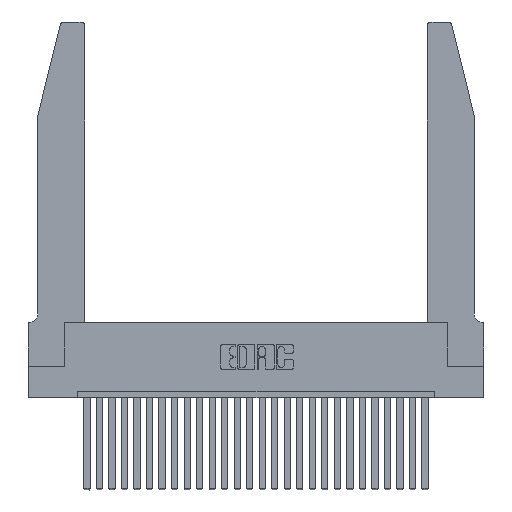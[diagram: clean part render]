
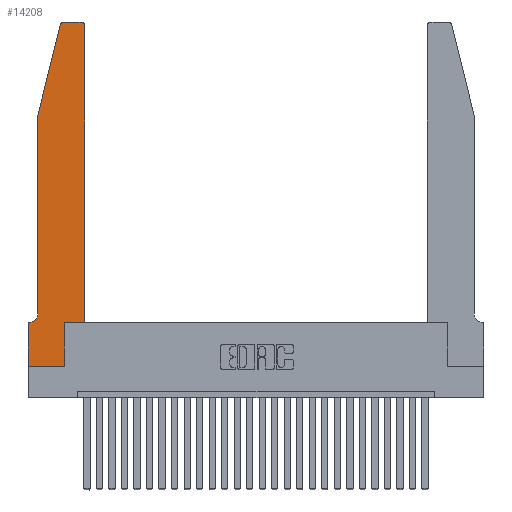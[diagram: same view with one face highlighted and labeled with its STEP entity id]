
A CAD part, top view. The second image highlights one B-rep face of the part: STEP entity #14208.
In plain terms, the highlighted planar face has unit normal (0, 0, 1).
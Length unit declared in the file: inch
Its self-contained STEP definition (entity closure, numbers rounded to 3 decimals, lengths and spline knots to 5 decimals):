
#185 = DIRECTION ( 'NONE',  ( 1., 0., 0. ) ) ;
#214 = ORIENTED_EDGE ( 'NONE', *, *, #17555, .T. ) ;
#443 = VECTOR ( 'NONE', #8880, 39.37008 ) ;
#586 = CARTESIAN_POINT ( 'NONE',  ( 0.2605, 2.75, 0.37 ) ) ;
#982 = EDGE_CURVE ( 'NONE', #19145, #22454, #14397, .T. ) ;
#1420 = EDGE_CURVE ( 'NONE', #19592, #8688, #21034, .T. ) ;
#1856 = AXIS2_PLACEMENT_3D ( 'NONE', #17353, #21535, #23645 ) ;
#1897 = CARTESIAN_POINT ( 'NONE',  ( 0.2865, 0.35, 0.37 ) ) ;
#2103 = CARTESIAN_POINT ( 'NONE',  ( 0.0055, 0.35, 0.37 ) ) ;
#2295 = VECTOR ( 'NONE', #12975, 39.37008 ) ;
#2397 = FACE_OUTER_BOUND ( 'NONE', #25852, .T. ) ;
#3489 = ORIENTED_EDGE ( 'NONE', *, *, #18303, .T. ) ;
#3810 = CIRCLE ( 'NONE', #1856, 0.03 ) ;
#4190 = LINE ( 'NONE', #22873, #16880 ) ;
#4228 = EDGE_CURVE ( 'NONE', #26464, #13652, #11018, .T. ) ;
#4322 = CARTESIAN_POINT ( 'NONE',  ( 0.4205, 2.75, 0.37 ) ) ;
#4453 = ORIENTED_EDGE ( 'NONE', *, *, #21800, .T. ) ;
#4820 = DIRECTION ( 'NONE',  ( -1., 0., 0. ) ) ;
#4891 = ORIENTED_EDGE ( 'NONE', *, *, #11842, .T. ) ;
#4965 = DIRECTION ( 'NONE',  ( 0., 1., 0. ) ) ;
#5534 = CARTESIAN_POINT ( 'NONE',  ( 0.4505, 2.72, 0.37 ) ) ;
#6410 = CARTESIAN_POINT ( 'NONE',  ( 0., 0., 0.37 ) ) ;
#6593 = CARTESIAN_POINT ( 'NONE',  ( 0.0755, 2., 0.37 ) ) ;
#6822 = LINE ( 'NONE', #22109, #26061 ) ;
#6920 = CIRCLE ( 'NONE', #12871, 0.07 ) ;
#7059 = EDGE_CURVE ( 'NONE', #15594, #19592, #4190, .T. ) ;
#7537 = LINE ( 'NONE', #1897, #22514 ) ;
#7857 = CARTESIAN_POINT ( 'NONE',  ( 0.4205, 2.72, 0.37 ) ) ;
#8307 = VERTEX_POINT ( 'NONE', #15370 ) ;
#8688 = VERTEX_POINT ( 'NONE', #20620 ) ;
#8880 = DIRECTION ( 'NONE',  ( -1., 0., 0. ) ) ;
#9003 = ORIENTED_EDGE ( 'NONE', *, *, #1420, .T. ) ;
#9033 = PLANE ( 'NONE',  #21551 ) ;
#9568 = LINE ( 'NONE', #10798, #11600 ) ;
#10331 = EDGE_CURVE ( 'NONE', #17383, #26464, #17255, .T. ) ;
#10453 = CARTESIAN_POINT ( 'NONE',  ( 0.2865, 0.35, 0.37 ) ) ;
#10753 = DIRECTION ( 'NONE',  ( 0., -1., 0. ) ) ;
#10798 = CARTESIAN_POINT ( 'NONE',  ( 0.4505, 0.35, 0.37 ) ) ;
#11018 = LINE ( 'NONE', #586, #25864 ) ;
#11600 = VECTOR ( 'NONE', #185, 39.37008 ) ;
#11688 = CARTESIAN_POINT ( 'NONE',  ( 0., 0.35, 0.37 ) ) ;
#11842 = EDGE_CURVE ( 'NONE', #8688, #12333, #7537, .T. ) ;
#11906 = DIRECTION ( 'NONE',  ( 0., 0., 1. ) ) ;
#12333 = VERTEX_POINT ( 'NONE', #10453 ) ;
#12681 = LINE ( 'NONE', #19303, #2295 ) ;
#12753 = VECTOR ( 'NONE', #10753, 39.37008 ) ;
#12871 = AXIS2_PLACEMENT_3D ( 'NONE', #15538, #19623, #23682 ) ;
#12975 = DIRECTION ( 'NONE',  ( -0.239, -0.971, 0. ) ) ;
#13126 = DIRECTION ( 'NONE',  ( 0., 0., 1. ) ) ;
#13652 = VERTEX_POINT ( 'NONE', #23832 ) ;
#13680 = CARTESIAN_POINT ( 'NONE',  ( 0.0755, 2., 0.37 ) ) ;
#14208 = ADVANCED_FACE ( 'NONE', ( #2397 ), #9033, .T. ) ;
#14397 = LINE ( 'NONE', #6593, #12753 ) ;
#14686 = DIRECTION ( 'NONE',  ( 0., 1., 0. ) ) ;
#15370 = CARTESIAN_POINT ( 'NONE',  ( 0.4505, 0.35, 0.37 ) ) ;
#15371 = VECTOR ( 'NONE', #18825, 39.37008 ) ;
#15538 = CARTESIAN_POINT ( 'NONE',  ( 0.0055, 0.42, 0.37 ) ) ;
#15594 = VERTEX_POINT ( 'NONE', #11688 ) ;
#15820 = EDGE_CURVE ( 'NONE', #22454, #16036, #6920, .T. ) ;
#16036 = VERTEX_POINT ( 'NONE', #2103 ) ;
#16338 = DIRECTION ( 'NONE',  ( 1., 0., 0. ) ) ;
#16537 = AXIS2_PLACEMENT_3D ( 'NONE', #7857, #11906, #16338 ) ;
#16880 = VECTOR ( 'NONE', #22963, 39.37008 ) ;
#17255 = CIRCLE ( 'NONE', #16537, 0.03 ) ;
#17298 = DIRECTION ( 'NONE',  ( 1., 0., 0. ) ) ;
#17353 = CARTESIAN_POINT ( 'NONE',  ( 0.284, 2.72, 0.37 ) ) ;
#17383 = VERTEX_POINT ( 'NONE', #5534 ) ;
#17555 = EDGE_CURVE ( 'NONE', #8307, #17383, #6822, .T. ) ;
#17819 = ORIENTED_EDGE ( 'NONE', *, *, #982, .T. ) ;
#17975 = CARTESIAN_POINT ( 'NONE',  ( 0.25487, 2.72718, 0.37 ) ) ;
#18303 = EDGE_CURVE ( 'NONE', #16036, #15594, #18473, .T. ) ;
#18473 = LINE ( 'NONE', #19433, #443 ) ;
#18825 = DIRECTION ( 'NONE',  ( 1., 0., 0. ) ) ;
#19145 = VERTEX_POINT ( 'NONE', #13680 ) ;
#19303 = CARTESIAN_POINT ( 'NONE',  ( 0.0755, 2., 0.37 ) ) ;
#19433 = CARTESIAN_POINT ( 'NONE',  ( 0.0755, 0.35, 0.37 ) ) ;
#19592 = VERTEX_POINT ( 'NONE', #24529 ) ;
#19617 = CARTESIAN_POINT ( 'NONE',  ( 0., 0.35, 0.37 ) ) ;
#19623 = DIRECTION ( 'NONE',  ( 0., 0., -1. ) ) ;
#20620 = CARTESIAN_POINT ( 'NONE',  ( 0.2865, 0., 0.37 ) ) ;
#20985 = ORIENTED_EDGE ( 'NONE', *, *, #7059, .T. ) ;
#21034 = LINE ( 'NONE', #6410, #15371 ) ;
#21535 = DIRECTION ( 'NONE',  ( 0., 0., 1. ) ) ;
#21551 = AXIS2_PLACEMENT_3D ( 'NONE', #19617, #13126, #17298 ) ;
#21681 = CARTESIAN_POINT ( 'NONE',  ( 0.0755, 0.42, 0.37 ) ) ;
#21800 = EDGE_CURVE ( 'NONE', #13652, #26780, #3810, .T. ) ;
#22109 = CARTESIAN_POINT ( 'NONE',  ( 0.4505, 0.35, 0.37 ) ) ;
#22454 = VERTEX_POINT ( 'NONE', #21681 ) ;
#22514 = VECTOR ( 'NONE', #14686, 39.37008 ) ;
#22873 = CARTESIAN_POINT ( 'NONE',  ( 0., 0., 0.37 ) ) ;
#22963 = DIRECTION ( 'NONE',  ( 0., -1., 0. ) ) ;
#23157 = ORIENTED_EDGE ( 'NONE', *, *, #15820, .T. ) ;
#23645 = DIRECTION ( 'NONE',  ( 1., 0., 0. ) ) ;
#23682 = DIRECTION ( 'NONE',  ( -1., 0., 0. ) ) ;
#23832 = CARTESIAN_POINT ( 'NONE',  ( 0.284, 2.75, 0.37 ) ) ;
#23944 = ORIENTED_EDGE ( 'NONE', *, *, #4228, .T. ) ;
#24529 = CARTESIAN_POINT ( 'NONE',  ( 0., 0., 0.37 ) ) ;
#24920 = ORIENTED_EDGE ( 'NONE', *, *, #26446, .T. ) ;
#25077 = ORIENTED_EDGE ( 'NONE', *, *, #10331, .T. ) ;
#25296 = EDGE_CURVE ( 'NONE', #26780, #19145, #12681, .T. ) ;
#25852 = EDGE_LOOP ( 'NONE', ( #23944, #4453, #26392, #17819, #23157, #3489, #20985, #9003, #4891, #24920, #214, #25077 ) ) ;
#25864 = VECTOR ( 'NONE', #4820, 39.37008 ) ;
#26061 = VECTOR ( 'NONE', #4965, 39.37008 ) ;
#26392 = ORIENTED_EDGE ( 'NONE', *, *, #25296, .T. ) ;
#26446 = EDGE_CURVE ( 'NONE', #12333, #8307, #9568, .T. ) ;
#26464 = VERTEX_POINT ( 'NONE', #4322 ) ;
#26780 = VERTEX_POINT ( 'NONE', #17975 ) ;
